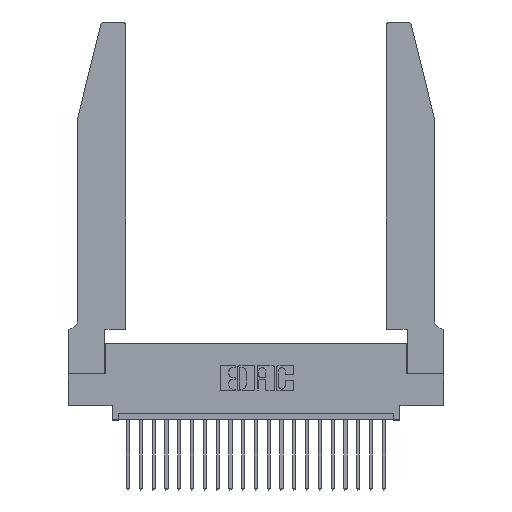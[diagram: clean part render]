
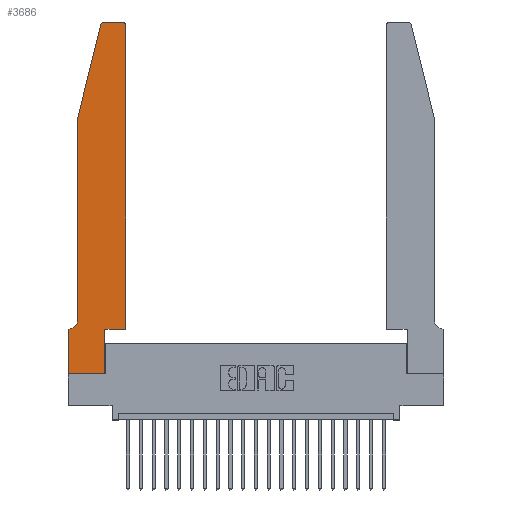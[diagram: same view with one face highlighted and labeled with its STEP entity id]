
A CAD part, top view. The second image highlights one B-rep face of the part: STEP entity #3686.
In plain terms, the highlighted planar face has unit normal (0, 0, 1).
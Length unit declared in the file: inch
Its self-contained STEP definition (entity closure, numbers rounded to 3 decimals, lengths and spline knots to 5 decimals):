
#19 = VERTEX_POINT ( 'NONE', #18486 ) ;
#131 = DIRECTION ( 'NONE',  ( -1., 0., 0. ) ) ;
#140 = DIRECTION ( 'NONE',  ( 0., 0., 1. ) ) ;
#524 = VERTEX_POINT ( 'NONE', #20466 ) ;
#644 = ORIENTED_EDGE ( 'NONE', *, *, #21930, .T. ) ;
#676 = CARTESIAN_POINT ( 'NONE',  ( 0.4505, 0.35, 0.37 ) ) ;
#750 = LINE ( 'NONE', #3704, #6168 ) ;
#1036 = CARTESIAN_POINT ( 'NONE',  ( 0.0755, 2., 0.37 ) ) ;
#1094 = ORIENTED_EDGE ( 'NONE', *, *, #23021, .T. ) ;
#1213 = DIRECTION ( 'NONE',  ( -1., 0., 0. ) ) ;
#1767 = VECTOR ( 'NONE', #20632, 39.37008 ) ;
#1930 = CARTESIAN_POINT ( 'NONE',  ( 0.2865, 0.35, 0.37 ) ) ;
#2023 = EDGE_CURVE ( 'NONE', #10792, #18609, #21046, .T. ) ;
#2295 = AXIS2_PLACEMENT_3D ( 'NONE', #21296, #12006, #1213 ) ;
#2318 = EDGE_CURVE ( 'NONE', #18609, #16236, #5504, .T. ) ;
#2778 = CIRCLE ( 'NONE', #16252, 0.03 ) ;
#2861 = VECTOR ( 'NONE', #14603, 39.37008 ) ;
#3087 = EDGE_LOOP ( 'NONE', ( #23388, #15204, #19998, #644, #1094, #20305, #13057, #8314, #3104, #13483, #16617, #8153 ) ) ;
#3104 = ORIENTED_EDGE ( 'NONE', *, *, #2023, .T. ) ;
#3686 = ADVANCED_FACE ( 'NONE', ( #14250 ), #4287, .T. ) ;
#3704 = CARTESIAN_POINT ( 'NONE',  ( 0.0755, 0.35, 0.37 ) ) ;
#4287 = PLANE ( 'NONE',  #13411 ) ;
#4527 = CARTESIAN_POINT ( 'NONE',  ( 0.4505, 0.35, 0.37 ) ) ;
#4801 = VERTEX_POINT ( 'NONE', #6119 ) ;
#5216 = VECTOR ( 'NONE', #13781, 39.37008 ) ;
#5504 = LINE ( 'NONE', #4527, #5216 ) ;
#5684 = CARTESIAN_POINT ( 'NONE',  ( 0.0755, 0.42, 0.37 ) ) ;
#6119 = CARTESIAN_POINT ( 'NONE',  ( 0.4505, 2.72, 0.37 ) ) ;
#6133 = DIRECTION ( 'NONE',  ( 1., 0., 0. ) ) ;
#6168 = VECTOR ( 'NONE', #131, 39.37008 ) ;
#6284 = CIRCLE ( 'NONE', #17814, 0.03 ) ;
#6798 = CARTESIAN_POINT ( 'NONE',  ( 0., 0., 0.37 ) ) ;
#6903 = EDGE_CURVE ( 'NONE', #22982, #524, #23507, .T. ) ;
#6941 = EDGE_CURVE ( 'NONE', #4801, #22982, #2778, .T. ) ;
#7425 = DIRECTION ( 'NONE',  ( 0., 1., 0. ) ) ;
#7555 = CARTESIAN_POINT ( 'NONE',  ( 0.25487, 2.72718, 0.37 ) ) ;
#7861 = DIRECTION ( 'NONE',  ( 0., 0., 1. ) ) ;
#8149 = DIRECTION ( 'NONE',  ( -1., 0., 0. ) ) ;
#8153 = ORIENTED_EDGE ( 'NONE', *, *, #6941, .T. ) ;
#8314 = ORIENTED_EDGE ( 'NONE', *, *, #21209, .T. ) ;
#8515 = CIRCLE ( 'NONE', #2295, 0.07 ) ;
#8557 = CARTESIAN_POINT ( 'NONE',  ( 0.284, 2.72, 0.37 ) ) ;
#8738 = VECTOR ( 'NONE', #8149, 39.37008 ) ;
#8868 = VECTOR ( 'NONE', #21395, 39.37008 ) ;
#8928 = VERTEX_POINT ( 'NONE', #18902 ) ;
#9929 = EDGE_CURVE ( 'NONE', #524, #18573, #6284, .T. ) ;
#10000 = CARTESIAN_POINT ( 'NONE',  ( 0., 0., 0.37 ) ) ;
#10372 = DIRECTION ( 'NONE',  ( 0., 0., 1. ) ) ;
#10792 = VERTEX_POINT ( 'NONE', #20378 ) ;
#10864 = DIRECTION ( 'NONE',  ( 1., 0., 0. ) ) ;
#10929 = LINE ( 'NONE', #10998, #13185 ) ;
#10998 = CARTESIAN_POINT ( 'NONE',  ( 0.4505, 0.35, 0.37 ) ) ;
#11789 = VERTEX_POINT ( 'NONE', #16640 ) ;
#12006 = DIRECTION ( 'NONE',  ( 0., 0., -1. ) ) ;
#12414 = EDGE_CURVE ( 'NONE', #8928, #11789, #750, .T. ) ;
#13057 = ORIENTED_EDGE ( 'NONE', *, *, #21097, .T. ) ;
#13185 = VECTOR ( 'NONE', #7425, 39.37008 ) ;
#13282 = CARTESIAN_POINT ( 'NONE',  ( 0.0755, 2., 0.37 ) ) ;
#13411 = AXIS2_PLACEMENT_3D ( 'NONE', #16963, #7861, #6133 ) ;
#13417 = VECTOR ( 'NONE', #22888, 39.37008 ) ;
#13483 = ORIENTED_EDGE ( 'NONE', *, *, #2318, .T. ) ;
#13667 = LINE ( 'NONE', #10000, #8868 ) ;
#13710 = CARTESIAN_POINT ( 'NONE',  ( 0.2865, 0.35, 0.37 ) ) ;
#13781 = DIRECTION ( 'NONE',  ( 1., 0., 0. ) ) ;
#13981 = LINE ( 'NONE', #1036, #13417 ) ;
#14250 = FACE_OUTER_BOUND ( 'NONE', #3087, .T. ) ;
#14330 = CARTESIAN_POINT ( 'NONE',  ( 0.4205, 2.72, 0.37 ) ) ;
#14603 = DIRECTION ( 'NONE',  ( 0., 1., 0. ) ) ;
#15005 = CARTESIAN_POINT ( 'NONE',  ( 0.4205, 2.75, 0.37 ) ) ;
#15204 = ORIENTED_EDGE ( 'NONE', *, *, #9929, .T. ) ;
#15678 = LINE ( 'NONE', #16483, #21091 ) ;
#16236 = VERTEX_POINT ( 'NONE', #676 ) ;
#16252 = AXIS2_PLACEMENT_3D ( 'NONE', #14330, #140, #10864 ) ;
#16483 = CARTESIAN_POINT ( 'NONE',  ( 0., 0., 0.37 ) ) ;
#16617 = ORIENTED_EDGE ( 'NONE', *, *, #19258, .T. ) ;
#16640 = CARTESIAN_POINT ( 'NONE',  ( 0., 0.35, 0.37 ) ) ;
#16815 = LINE ( 'NONE', #13282, #1767 ) ;
#16963 = CARTESIAN_POINT ( 'NONE',  ( 0., 0.35, 0.37 ) ) ;
#17167 = CARTESIAN_POINT ( 'NONE',  ( 0.2605, 2.75, 0.37 ) ) ;
#17814 = AXIS2_PLACEMENT_3D ( 'NONE', #8557, #10372, #21256 ) ;
#18486 = CARTESIAN_POINT ( 'NONE',  ( 0.0755, 2., 0.37 ) ) ;
#18573 = VERTEX_POINT ( 'NONE', #7555 ) ;
#18609 = VERTEX_POINT ( 'NONE', #13710 ) ;
#18902 = CARTESIAN_POINT ( 'NONE',  ( 0.0055, 0.35, 0.37 ) ) ;
#19164 = VERTEX_POINT ( 'NONE', #5684 ) ;
#19258 = EDGE_CURVE ( 'NONE', #16236, #4801, #10929, .T. ) ;
#19998 = ORIENTED_EDGE ( 'NONE', *, *, #20664, .T. ) ;
#20016 = DIRECTION ( 'NONE',  ( 0., -1., 0. ) ) ;
#20305 = ORIENTED_EDGE ( 'NONE', *, *, #12414, .T. ) ;
#20378 = CARTESIAN_POINT ( 'NONE',  ( 0.2865, 0., 0.37 ) ) ;
#20466 = CARTESIAN_POINT ( 'NONE',  ( 0.284, 2.75, 0.37 ) ) ;
#20632 = DIRECTION ( 'NONE',  ( 0., -1., 0. ) ) ;
#20664 = EDGE_CURVE ( 'NONE', #18573, #19, #13981, .T. ) ;
#21046 = LINE ( 'NONE', #1930, #2861 ) ;
#21091 = VECTOR ( 'NONE', #20016, 39.37008 ) ;
#21097 = EDGE_CURVE ( 'NONE', #11789, #22807, #15678, .T. ) ;
#21209 = EDGE_CURVE ( 'NONE', #22807, #10792, #13667, .T. ) ;
#21256 = DIRECTION ( 'NONE',  ( 1., 0., 0. ) ) ;
#21296 = CARTESIAN_POINT ( 'NONE',  ( 0.0055, 0.42, 0.37 ) ) ;
#21395 = DIRECTION ( 'NONE',  ( 1., 0., 0. ) ) ;
#21930 = EDGE_CURVE ( 'NONE', #19, #19164, #16815, .T. ) ;
#22807 = VERTEX_POINT ( 'NONE', #6798 ) ;
#22888 = DIRECTION ( 'NONE',  ( -0.239, -0.971, 0. ) ) ;
#22982 = VERTEX_POINT ( 'NONE', #15005 ) ;
#23021 = EDGE_CURVE ( 'NONE', #19164, #8928, #8515, .T. ) ;
#23388 = ORIENTED_EDGE ( 'NONE', *, *, #6903, .T. ) ;
#23507 = LINE ( 'NONE', #17167, #8738 ) ;
